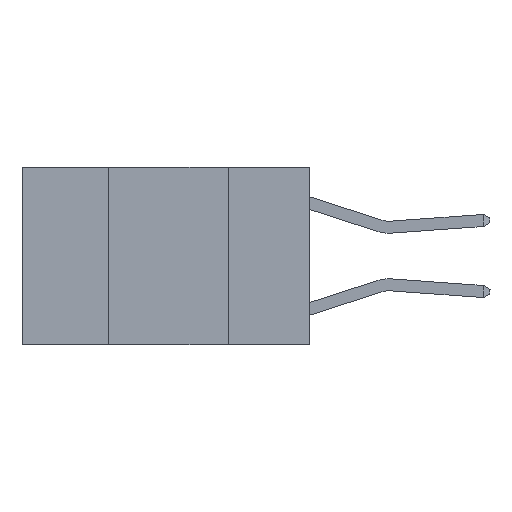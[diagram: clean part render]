
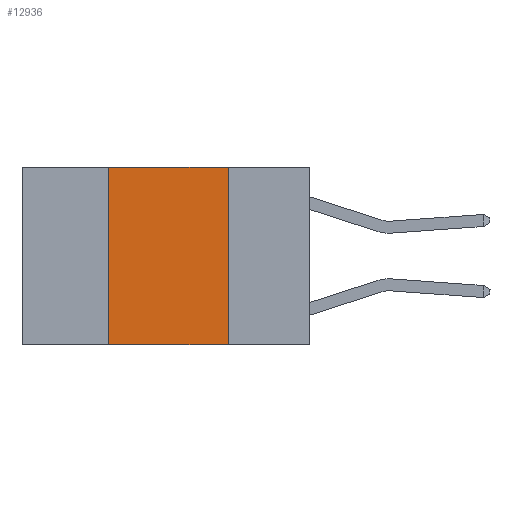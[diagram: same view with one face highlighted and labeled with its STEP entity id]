
A CAD part, left-side view. The second image highlights one B-rep face of the part: STEP entity #12936.
In plain terms, the highlighted planar face has unit normal (-1, 0, 0).
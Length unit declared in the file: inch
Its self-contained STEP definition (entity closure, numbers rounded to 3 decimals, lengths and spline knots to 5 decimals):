
#498 = EDGE_CURVE ( 'NONE', #8148, #12529, #8799, .T. ) ;
#1597 = EDGE_CURVE ( 'NONE', #4609, #10133, #4899, .T. ) ;
#1740 = PLANE ( 'NONE',  #11511 ) ;
#1781 = CARTESIAN_POINT ( 'NONE',  ( 0., 0.6, 0. ) ) ;
#1809 = ORIENTED_EDGE ( 'NONE', *, *, #15333, .F. ) ;
#2212 = DIRECTION ( 'NONE',  ( 0., 0., 1. ) ) ;
#3161 = CARTESIAN_POINT ( 'NONE',  ( 0., 0.17, 0. ) ) ;
#4248 = CARTESIAN_POINT ( 'NONE',  ( 0., 0.17, 0. ) ) ;
#4609 = VERTEX_POINT ( 'NONE', #8094 ) ;
#4899 = LINE ( 'NONE', #13129, #16644 ) ;
#5631 = CARTESIAN_POINT ( 'NONE',  ( 0., 0.6, 0. ) ) ;
#6596 = CARTESIAN_POINT ( 'NONE',  ( 0., 0.17, -0.37 ) ) ;
#7085 = FACE_OUTER_BOUND ( 'NONE', #13175, .T. ) ;
#7253 = DIRECTION ( 'NONE',  ( 0., 0., -1. ) ) ;
#7845 = CARTESIAN_POINT ( 'NONE',  ( 0., 0.42, 0. ) ) ;
#8094 = CARTESIAN_POINT ( 'NONE',  ( 0., 0.42, -0.37 ) ) ;
#8148 = VERTEX_POINT ( 'NONE', #7845 ) ;
#8386 = VECTOR ( 'NONE', #2212, 39.37008 ) ;
#8448 = EDGE_CURVE ( 'NONE', #12529, #10133, #11744, .T. ) ;
#8799 = LINE ( 'NONE', #1781, #10847 ) ;
#9158 = VECTOR ( 'NONE', #14348, 39.37008 ) ;
#10133 = VERTEX_POINT ( 'NONE', #6596 ) ;
#10847 = VECTOR ( 'NONE', #12742, 39.37008 ) ;
#11511 = AXIS2_PLACEMENT_3D ( 'NONE', #5631, #12532, #7253 ) ;
#11720 = LINE ( 'NONE', #17194, #8386 ) ;
#11744 = LINE ( 'NONE', #3161, #9158 ) ;
#11769 = DIRECTION ( 'NONE',  ( 0., -1., 0. ) ) ;
#12529 = VERTEX_POINT ( 'NONE', #4248 ) ;
#12532 = DIRECTION ( 'NONE',  ( 1., 0., 0. ) ) ;
#12742 = DIRECTION ( 'NONE',  ( 0., -1., 0. ) ) ;
#12936 = ADVANCED_FACE ( 'NONE', ( #7085 ), #1740, .F. ) ;
#13129 = CARTESIAN_POINT ( 'NONE',  ( 0., 0.6, -0.37 ) ) ;
#13175 = EDGE_LOOP ( 'NONE', ( #14392, #16547, #1809, #17293 ) ) ;
#14348 = DIRECTION ( 'NONE',  ( 0., 0., -1. ) ) ;
#14392 = ORIENTED_EDGE ( 'NONE', *, *, #8448, .F. ) ;
#15333 = EDGE_CURVE ( 'NONE', #4609, #8148, #11720, .T. ) ;
#16547 = ORIENTED_EDGE ( 'NONE', *, *, #498, .F. ) ;
#16644 = VECTOR ( 'NONE', #11769, 39.37008 ) ;
#17194 = CARTESIAN_POINT ( 'NONE',  ( 0., 0.42, 0. ) ) ;
#17293 = ORIENTED_EDGE ( 'NONE', *, *, #1597, .T. ) ;
